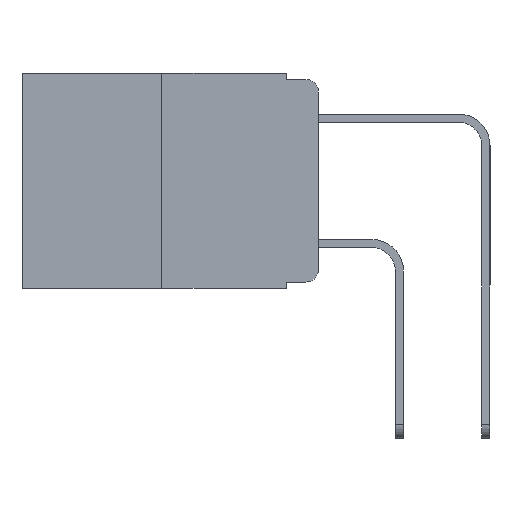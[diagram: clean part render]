
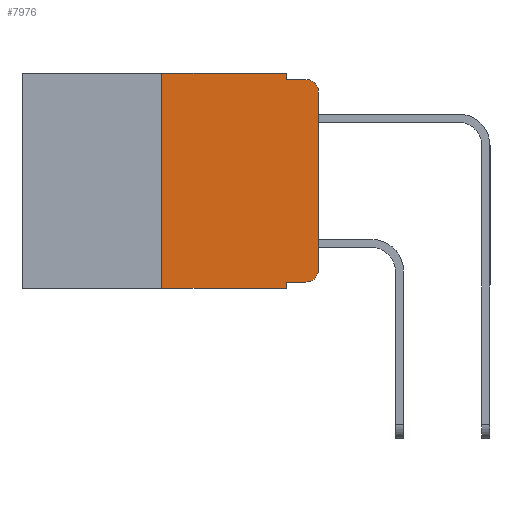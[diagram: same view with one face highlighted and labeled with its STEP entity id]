
A CAD part, left-side view. The second image highlights one B-rep face of the part: STEP entity #7976.
In plain terms, the highlighted planar face has unit normal (-1, 0, 0).
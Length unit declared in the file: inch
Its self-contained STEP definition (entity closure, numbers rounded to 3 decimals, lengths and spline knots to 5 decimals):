
#145 = PLANE ( 'NONE',  #5662 ) ;
#261 = LINE ( 'NONE', #7092, #4046 ) ;
#814 = VERTEX_POINT ( 'NONE', #16472 ) ;
#952 = CARTESIAN_POINT ( 'NONE',  ( 0., 0.02, -0.313 ) ) ;
#990 = VERTEX_POINT ( 'NONE', #9055 ) ;
#1134 = CARTESIAN_POINT ( 'NONE',  ( 0., 0., 0. ) ) ;
#1319 = FACE_OUTER_BOUND ( 'NONE', #3617, .T. ) ;
#1457 = LINE ( 'NONE', #8613, #4345 ) ;
#1539 = VERTEX_POINT ( 'NONE', #16915 ) ;
#1566 = DIRECTION ( 'NONE',  ( 1., 0., 0. ) ) ;
#1651 = VECTOR ( 'NONE', #9429, 39.37008 ) ;
#1817 = ORIENTED_EDGE ( 'NONE', *, *, #13109, .T. ) ;
#2306 = EDGE_CURVE ( 'NONE', #1539, #6711, #5646, .T. ) ;
#2412 = DIRECTION ( 'NONE',  ( 0., 0., -1. ) ) ;
#2968 = CARTESIAN_POINT ( 'NONE',  ( 0., 0.473, 0. ) ) ;
#3197 = VERTEX_POINT ( 'NONE', #10430 ) ;
#3339 = VERTEX_POINT ( 'NONE', #11424 ) ;
#3386 = ORIENTED_EDGE ( 'NONE', *, *, #7064, .F. ) ;
#3617 = EDGE_LOOP ( 'NONE', ( #4445, #7948, #8343, #15129, #15895, #3386, #6907, #10786, #1817, #15722 ) ) ;
#3714 = VECTOR ( 'NONE', #11074, 39.37008 ) ;
#4046 = VECTOR ( 'NONE', #14766, 39.37008 ) ;
#4262 = CIRCLE ( 'NONE', #12044, 0.02 ) ;
#4298 = VERTEX_POINT ( 'NONE', #15957 ) ;
#4345 = VECTOR ( 'NONE', #16211, 39.37008 ) ;
#4445 = ORIENTED_EDGE ( 'NONE', *, *, #15725, .T. ) ;
#4711 = CARTESIAN_POINT ( 'NONE',  ( 0., 0.473, -0.343 ) ) ;
#5127 = CARTESIAN_POINT ( 'NONE',  ( 0., 0.051, -0.01 ) ) ;
#5243 = VECTOR ( 'NONE', #6947, 39.37008 ) ;
#5314 = EDGE_CURVE ( 'NONE', #3339, #1539, #5347, .T. ) ;
#5331 = DIRECTION ( 'NONE',  ( -1., 0., 0. ) ) ;
#5347 = LINE ( 'NONE', #16106, #1651 ) ;
#5442 = VERTEX_POINT ( 'NONE', #9156 ) ;
#5466 = CARTESIAN_POINT ( 'NONE',  ( 0., 0.473, 0. ) ) ;
#5646 = LINE ( 'NONE', #5127, #5243 ) ;
#5662 = AXIS2_PLACEMENT_3D ( 'NONE', #2968, #1566, #10925 ) ;
#6007 = VERTEX_POINT ( 'NONE', #11167 ) ;
#6586 = VECTOR ( 'NONE', #16262, 39.37008 ) ;
#6711 = VERTEX_POINT ( 'NONE', #12687 ) ;
#6766 = DIRECTION ( 'NONE',  ( 0., -1., 0. ) ) ;
#6907 = ORIENTED_EDGE ( 'NONE', *, *, #10522, .T. ) ;
#6947 = DIRECTION ( 'NONE',  ( 0., -1., 0. ) ) ;
#7064 = EDGE_CURVE ( 'NONE', #990, #5442, #261, .T. ) ;
#7092 = CARTESIAN_POINT ( 'NONE',  ( 0., 0.25, 0. ) ) ;
#7948 = ORIENTED_EDGE ( 'NONE', *, *, #16550, .T. ) ;
#7965 = VECTOR ( 'NONE', #6766, 39.37008 ) ;
#7976 = ADVANCED_FACE ( 'NONE', ( #1319 ), #145, .F. ) ;
#8343 = ORIENTED_EDGE ( 'NONE', *, *, #2306, .F. ) ;
#8460 = CARTESIAN_POINT ( 'NONE',  ( 0., 0.051, 0. ) ) ;
#8613 = CARTESIAN_POINT ( 'NONE',  ( 0., 0.051, -0.333 ) ) ;
#9055 = CARTESIAN_POINT ( 'NONE',  ( 0., 0.25, -0.343 ) ) ;
#9156 = CARTESIAN_POINT ( 'NONE',  ( 0., 0.25, 0. ) ) ;
#9429 = DIRECTION ( 'NONE',  ( 0., 0., -1. ) ) ;
#9580 = LINE ( 'NONE', #1134, #12585 ) ;
#9682 = EDGE_CURVE ( 'NONE', #14157, #814, #10688, .T. ) ;
#10057 = LINE ( 'NONE', #4711, #6586 ) ;
#10364 = DIRECTION ( 'NONE',  ( -1., 0., 0. ) ) ;
#10430 = CARTESIAN_POINT ( 'NONE',  ( 0., 0.02, -0.333 ) ) ;
#10522 = EDGE_CURVE ( 'NONE', #990, #814, #10057, .T. ) ;
#10688 = LINE ( 'NONE', #8460, #3714 ) ;
#10786 = ORIENTED_EDGE ( 'NONE', *, *, #9682, .F. ) ;
#10925 = DIRECTION ( 'NONE',  ( 0., 0., -1. ) ) ;
#11074 = DIRECTION ( 'NONE',  ( 0., 0., -1. ) ) ;
#11167 = CARTESIAN_POINT ( 'NONE',  ( 0., 0., -0.03 ) ) ;
#11424 = CARTESIAN_POINT ( 'NONE',  ( 0., 0.051, 0. ) ) ;
#11585 = CIRCLE ( 'NONE', #12560, 0.02 ) ;
#11835 = DIRECTION ( 'NONE',  ( 0., 0., 1. ) ) ;
#12044 = AXIS2_PLACEMENT_3D ( 'NONE', #952, #10364, #2412 ) ;
#12560 = AXIS2_PLACEMENT_3D ( 'NONE', #13065, #5331, #14341 ) ;
#12585 = VECTOR ( 'NONE', #11835, 39.37008 ) ;
#12687 = CARTESIAN_POINT ( 'NONE',  ( 0., 0.02, -0.01 ) ) ;
#13065 = CARTESIAN_POINT ( 'NONE',  ( 0., 0.02, -0.03 ) ) ;
#13109 = EDGE_CURVE ( 'NONE', #14157, #3197, #1457, .T. ) ;
#14157 = VERTEX_POINT ( 'NONE', #15708 ) ;
#14341 = DIRECTION ( 'NONE',  ( 0., 0., -1. ) ) ;
#14766 = DIRECTION ( 'NONE',  ( 0., 0., 1. ) ) ;
#15129 = ORIENTED_EDGE ( 'NONE', *, *, #5314, .F. ) ;
#15535 = LINE ( 'NONE', #5466, #7965 ) ;
#15634 = EDGE_CURVE ( 'NONE', #3197, #4298, #4262, .T. ) ;
#15708 = CARTESIAN_POINT ( 'NONE',  ( 0., 0.051, -0.333 ) ) ;
#15722 = ORIENTED_EDGE ( 'NONE', *, *, #15634, .T. ) ;
#15725 = EDGE_CURVE ( 'NONE', #4298, #6007, #9580, .T. ) ;
#15813 = EDGE_CURVE ( 'NONE', #5442, #3339, #15535, .T. ) ;
#15895 = ORIENTED_EDGE ( 'NONE', *, *, #15813, .F. ) ;
#15957 = CARTESIAN_POINT ( 'NONE',  ( 0., 0., -0.313 ) ) ;
#16106 = CARTESIAN_POINT ( 'NONE',  ( 0., 0.051, 0. ) ) ;
#16211 = DIRECTION ( 'NONE',  ( 0., -1., 0. ) ) ;
#16262 = DIRECTION ( 'NONE',  ( 0., -1., 0. ) ) ;
#16472 = CARTESIAN_POINT ( 'NONE',  ( 0., 0.051, -0.343 ) ) ;
#16550 = EDGE_CURVE ( 'NONE', #6007, #6711, #11585, .T. ) ;
#16915 = CARTESIAN_POINT ( 'NONE',  ( 0., 0.051, -0.01 ) ) ;
